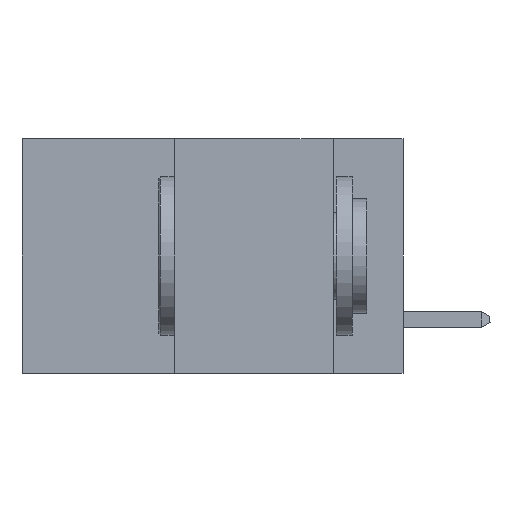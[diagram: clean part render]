
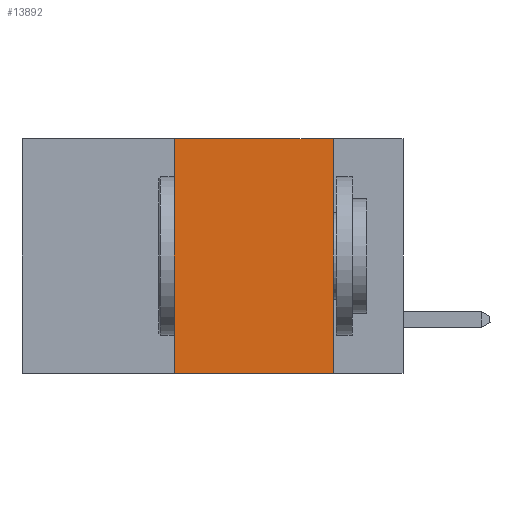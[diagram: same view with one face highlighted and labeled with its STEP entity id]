
A CAD part, left-side view. The second image highlights one B-rep face of the part: STEP entity #13892.
In plain terms, the highlighted planar face has unit normal (-1, 0, 0).
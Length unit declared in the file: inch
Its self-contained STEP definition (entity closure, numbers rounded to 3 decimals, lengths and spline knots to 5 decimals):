
#112 = CARTESIAN_POINT ( 'NONE',  ( 0., 0.36, 0. ) ) ;
#1852 = CARTESIAN_POINT ( 'NONE',  ( 0., 0.11, -0.37 ) ) ;
#1892 = ORIENTED_EDGE ( 'NONE', *, *, #21470, .F. ) ;
#3885 = DIRECTION ( 'NONE',  ( 0., 0., 1. ) ) ;
#4270 = CARTESIAN_POINT ( 'NONE',  ( 0., 0.6, 0. ) ) ;
#4508 = DIRECTION ( 'NONE',  ( 0., 0., -1. ) ) ;
#7645 = DIRECTION ( 'NONE',  ( 1., 0., 0. ) ) ;
#9909 = EDGE_CURVE ( 'NONE', #12307, #22802, #34108, .T. ) ;
#10262 = ORIENTED_EDGE ( 'NONE', *, *, #46699, .F. ) ;
#11887 = CARTESIAN_POINT ( 'NONE',  ( 0., 0.11, 0. ) ) ;
#12307 = VERTEX_POINT ( 'NONE', #46368 ) ;
#12327 = LINE ( 'NONE', #31461, #18186 ) ;
#13718 = FACE_OUTER_BOUND ( 'NONE', #43635, .T. ) ;
#13892 = ADVANCED_FACE ( 'NONE', ( #13718 ), #48183, .F. ) ;
#18186 = VECTOR ( 'NONE', #38675, 39.37008 ) ;
#21118 = LINE ( 'NONE', #4270, #28143 ) ;
#21470 = EDGE_CURVE ( 'NONE', #47193, #12307, #21118, .T. ) ;
#22802 = VERTEX_POINT ( 'NONE', #1852 ) ;
#23220 = DIRECTION ( 'NONE',  ( 0., -1., 0. ) ) ;
#24740 = EDGE_CURVE ( 'NONE', #26860, #22802, #12327, .T. ) ;
#25905 = CARTESIAN_POINT ( 'NONE',  ( 0., 0.36, 0. ) ) ;
#25948 = DIRECTION ( 'NONE',  ( 0., 0., -1. ) ) ;
#26860 = VERTEX_POINT ( 'NONE', #42956 ) ;
#28143 = VECTOR ( 'NONE', #23220, 39.37008 ) ;
#28435 = AXIS2_PLACEMENT_3D ( 'NONE', #29567, #7645, #25948 ) ;
#29567 = CARTESIAN_POINT ( 'NONE',  ( 0., 0.6, 0. ) ) ;
#31461 = CARTESIAN_POINT ( 'NONE',  ( 0., 0.6, -0.37 ) ) ;
#34021 = VECTOR ( 'NONE', #3885, 39.37008 ) ;
#34108 = LINE ( 'NONE', #11887, #37627 ) ;
#36708 = ORIENTED_EDGE ( 'NONE', *, *, #24740, .T. ) ;
#37231 = ORIENTED_EDGE ( 'NONE', *, *, #9909, .F. ) ;
#37627 = VECTOR ( 'NONE', #4508, 39.37008 ) ;
#38675 = DIRECTION ( 'NONE',  ( 0., -1., 0. ) ) ;
#42956 = CARTESIAN_POINT ( 'NONE',  ( 0., 0.36, -0.37 ) ) ;
#43635 = EDGE_LOOP ( 'NONE', ( #37231, #1892, #10262, #36708 ) ) ;
#45116 = LINE ( 'NONE', #112, #34021 ) ;
#46368 = CARTESIAN_POINT ( 'NONE',  ( 0., 0.11, 0. ) ) ;
#46699 = EDGE_CURVE ( 'NONE', #26860, #47193, #45116, .T. ) ;
#47193 = VERTEX_POINT ( 'NONE', #25905 ) ;
#48183 = PLANE ( 'NONE',  #28435 ) ;
